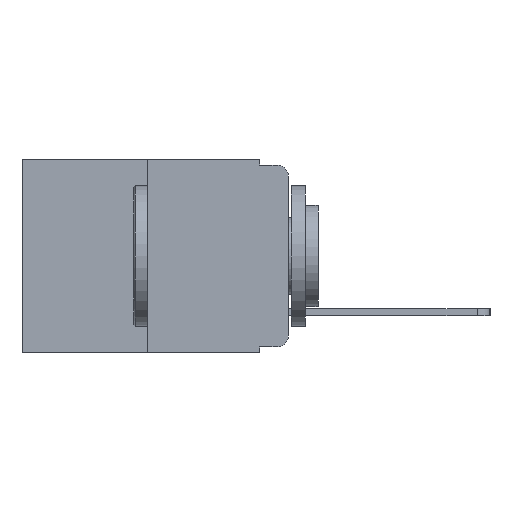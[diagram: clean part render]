
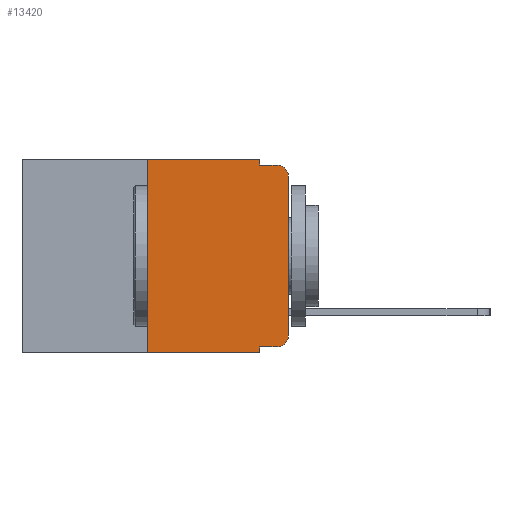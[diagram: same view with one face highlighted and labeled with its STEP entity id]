
A CAD part, left-side view. The second image highlights one B-rep face of the part: STEP entity #13420.
In plain terms, the highlighted planar face has unit normal (-1, 0, 0).
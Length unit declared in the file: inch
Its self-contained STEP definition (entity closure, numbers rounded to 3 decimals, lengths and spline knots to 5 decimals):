
#54 = CARTESIAN_POINT ( 'NONE',  ( 0., 0., -0.313 ) ) ;
#359 = DIRECTION ( 'NONE',  ( 0., -1., 0. ) ) ;
#706 = EDGE_CURVE ( 'NONE', #1657, #3573, #12114, .T. ) ;
#1037 = LINE ( 'NONE', #14976, #17607 ) ;
#1546 = EDGE_LOOP ( 'NONE', ( #8436, #4333, #14343, #3724, #17963, #13701, #1742, #10169, #11664, #17258 ) ) ;
#1657 = VERTEX_POINT ( 'NONE', #54 ) ;
#1742 = ORIENTED_EDGE ( 'NONE', *, *, #13891, .T. ) ;
#1994 = CARTESIAN_POINT ( 'NONE',  ( 0., 0.051, -0.01 ) ) ;
#2205 = LINE ( 'NONE', #16518, #6144 ) ;
#2392 = DIRECTION ( 'NONE',  ( 0., -1., 0. ) ) ;
#2770 = VECTOR ( 'NONE', #11888, 39.37008 ) ;
#3050 = LINE ( 'NONE', #15524, #11062 ) ;
#3573 = VERTEX_POINT ( 'NONE', #13400 ) ;
#3724 = ORIENTED_EDGE ( 'NONE', *, *, #5167, .F. ) ;
#3883 = EDGE_CURVE ( 'NONE', #3573, #4723, #15736, .T. ) ;
#3931 = DIRECTION ( 'NONE',  ( 0., 0., -1. ) ) ;
#4333 = ORIENTED_EDGE ( 'NONE', *, *, #3883, .T. ) ;
#4393 = AXIS2_PLACEMENT_3D ( 'NONE', #12444, #9329, #20144 ) ;
#4723 = VERTEX_POINT ( 'NONE', #16818 ) ;
#5167 = EDGE_CURVE ( 'NONE', #5622, #18291, #1037, .T. ) ;
#5622 = VERTEX_POINT ( 'NONE', #18400 ) ;
#5646 = AXIS2_PLACEMENT_3D ( 'NONE', #7521, #16867, #7686 ) ;
#6000 = EDGE_CURVE ( 'NONE', #7089, #1657, #10017, .T. ) ;
#6144 = VECTOR ( 'NONE', #359, 39.37008 ) ;
#6875 = DIRECTION ( 'NONE',  ( 0., 0., -1. ) ) ;
#7089 = VERTEX_POINT ( 'NONE', #8395 ) ;
#7161 = VERTEX_POINT ( 'NONE', #12088 ) ;
#7521 = CARTESIAN_POINT ( 'NONE',  ( 0., 0.02, -0.03 ) ) ;
#7686 = DIRECTION ( 'NONE',  ( 0., 0., -1. ) ) ;
#7701 = FACE_OUTER_BOUND ( 'NONE', #1546, .T. ) ;
#8395 = CARTESIAN_POINT ( 'NONE',  ( 0., 0.02, -0.333 ) ) ;
#8436 = ORIENTED_EDGE ( 'NONE', *, *, #706, .T. ) ;
#9329 = DIRECTION ( 'NONE',  ( 1., 0., 0. ) ) ;
#9470 = CARTESIAN_POINT ( 'NONE',  ( 0., 0.25, 0. ) ) ;
#9584 = CARTESIAN_POINT ( 'NONE',  ( 0., 0.25, 0. ) ) ;
#9843 = EDGE_CURVE ( 'NONE', #19504, #7161, #16772, .T. ) ;
#10017 = CIRCLE ( 'NONE', #11174, 0.02 ) ;
#10169 = ORIENTED_EDGE ( 'NONE', *, *, #9843, .F. ) ;
#10343 = CARTESIAN_POINT ( 'NONE',  ( 0., 0.473, 0. ) ) ;
#11062 = VECTOR ( 'NONE', #20053, 39.37008 ) ;
#11174 = AXIS2_PLACEMENT_3D ( 'NONE', #20553, #16644, #14959 ) ;
#11664 = ORIENTED_EDGE ( 'NONE', *, *, #13753, .T. ) ;
#11888 = DIRECTION ( 'NONE',  ( 0., -1., 0. ) ) ;
#12028 = CARTESIAN_POINT ( 'NONE',  ( 0., 0.051, -0.01 ) ) ;
#12088 = CARTESIAN_POINT ( 'NONE',  ( 0., 0.051, -0.343 ) ) ;
#12114 = LINE ( 'NONE', #15559, #16274 ) ;
#12444 = CARTESIAN_POINT ( 'NONE',  ( 0., 0.473, 0. ) ) ;
#12713 = CARTESIAN_POINT ( 'NONE',  ( 0., 0.051, -0.333 ) ) ;
#12768 = EDGE_CURVE ( 'NONE', #18291, #4723, #19824, .T. ) ;
#13016 = VERTEX_POINT ( 'NONE', #17328 ) ;
#13400 = CARTESIAN_POINT ( 'NONE',  ( 0., 0., -0.03 ) ) ;
#13420 = ADVANCED_FACE ( 'NONE', ( #7701 ), #18640, .F. ) ;
#13701 = ORIENTED_EDGE ( 'NONE', *, *, #15150, .F. ) ;
#13753 = EDGE_CURVE ( 'NONE', #19504, #7089, #2205, .T. ) ;
#13891 = EDGE_CURVE ( 'NONE', #13016, #7161, #3050, .T. ) ;
#14343 = ORIENTED_EDGE ( 'NONE', *, *, #12768, .F. ) ;
#14959 = DIRECTION ( 'NONE',  ( 0., 0., -1. ) ) ;
#14976 = CARTESIAN_POINT ( 'NONE',  ( 0., 0.051, 0. ) ) ;
#15150 = EDGE_CURVE ( 'NONE', #13016, #18767, #20604, .T. ) ;
#15258 = DIRECTION ( 'NONE',  ( 0., 0., 1. ) ) ;
#15524 = CARTESIAN_POINT ( 'NONE',  ( 0., 0.473, -0.343 ) ) ;
#15559 = CARTESIAN_POINT ( 'NONE',  ( 0., 0., 0. ) ) ;
#15736 = CIRCLE ( 'NONE', #5646, 0.02 ) ;
#15823 = VECTOR ( 'NONE', #3931, 39.37008 ) ;
#16274 = VECTOR ( 'NONE', #15258, 39.37008 ) ;
#16518 = CARTESIAN_POINT ( 'NONE',  ( 0., 0.051, -0.333 ) ) ;
#16644 = DIRECTION ( 'NONE',  ( -1., 0., 0. ) ) ;
#16759 = EDGE_CURVE ( 'NONE', #18767, #5622, #19512, .T. ) ;
#16772 = LINE ( 'NONE', #19568, #15823 ) ;
#16818 = CARTESIAN_POINT ( 'NONE',  ( 0., 0.02, -0.01 ) ) ;
#16867 = DIRECTION ( 'NONE',  ( -1., 0., 0. ) ) ;
#17258 = ORIENTED_EDGE ( 'NONE', *, *, #6000, .T. ) ;
#17328 = CARTESIAN_POINT ( 'NONE',  ( 0., 0.25, -0.343 ) ) ;
#17607 = VECTOR ( 'NONE', #6875, 39.37008 ) ;
#17963 = ORIENTED_EDGE ( 'NONE', *, *, #16759, .F. ) ;
#18291 = VERTEX_POINT ( 'NONE', #1994 ) ;
#18400 = CARTESIAN_POINT ( 'NONE',  ( 0., 0.051, 0. ) ) ;
#18640 = PLANE ( 'NONE',  #4393 ) ;
#18767 = VERTEX_POINT ( 'NONE', #9470 ) ;
#18878 = DIRECTION ( 'NONE',  ( 0., 0., 1. ) ) ;
#19504 = VERTEX_POINT ( 'NONE', #12713 ) ;
#19512 = LINE ( 'NONE', #10343, #2770 ) ;
#19568 = CARTESIAN_POINT ( 'NONE',  ( 0., 0.051, 0. ) ) ;
#19824 = LINE ( 'NONE', #12028, #20274 ) ;
#20053 = DIRECTION ( 'NONE',  ( 0., -1., 0. ) ) ;
#20144 = DIRECTION ( 'NONE',  ( 0., 0., -1. ) ) ;
#20147 = VECTOR ( 'NONE', #18878, 39.37008 ) ;
#20274 = VECTOR ( 'NONE', #2392, 39.37008 ) ;
#20553 = CARTESIAN_POINT ( 'NONE',  ( 0., 0.02, -0.313 ) ) ;
#20604 = LINE ( 'NONE', #9584, #20147 ) ;
